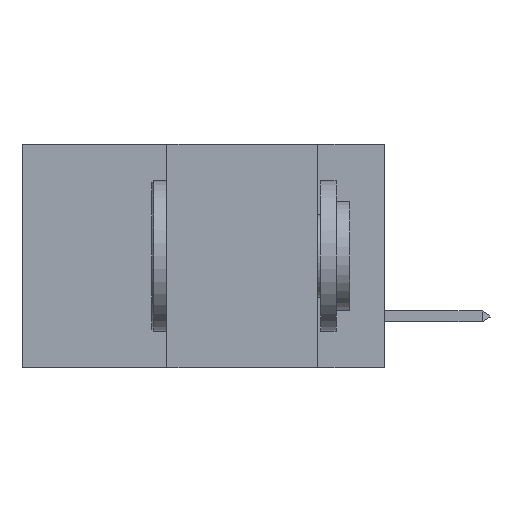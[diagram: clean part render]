
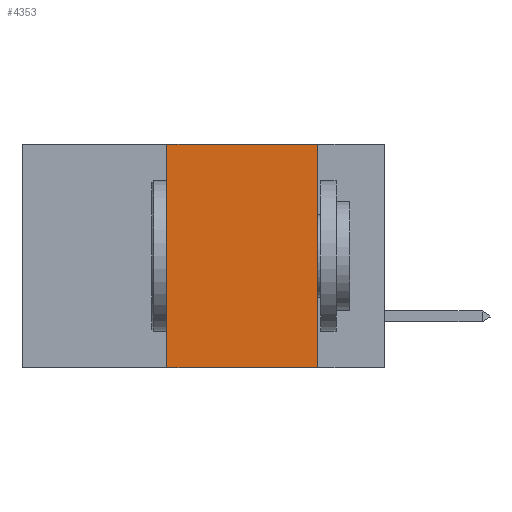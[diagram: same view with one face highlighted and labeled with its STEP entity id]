
A CAD part, left-side view. The second image highlights one B-rep face of the part: STEP entity #4353.
In plain terms, the highlighted planar face has unit normal (-1, 0, 0).
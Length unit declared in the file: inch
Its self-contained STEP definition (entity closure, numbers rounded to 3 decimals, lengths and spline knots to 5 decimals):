
#72 = CARTESIAN_POINT ( 'NONE',  ( 0., 0.11, -0.37 ) ) ;
#122 = CARTESIAN_POINT ( 'NONE',  ( 0., 0.36, -0.37 ) ) ;
#242 = CARTESIAN_POINT ( 'NONE',  ( 0., 0.36, 0. ) ) ;
#438 = CARTESIAN_POINT ( 'NONE',  ( 0., 0.11, 0. ) ) ;
#2073 = LINE ( 'NONE', #10217, #8807 ) ;
#2089 = ORIENTED_EDGE ( 'NONE', *, *, #7960, .F. ) ;
#2173 = PLANE ( 'NONE',  #8503 ) ;
#3237 = VECTOR ( 'NONE', #3608, 39.37008 ) ;
#3608 = DIRECTION ( 'NONE',  ( 0., -1., 0. ) ) ;
#3839 = LINE ( 'NONE', #12000, #12745 ) ;
#4127 = EDGE_CURVE ( 'NONE', #6710, #10587, #11072, .T. ) ;
#4353 = ADVANCED_FACE ( 'NONE', ( #7866 ), #2173, .F. ) ;
#4781 = VERTEX_POINT ( 'NONE', #72 ) ;
#5254 = VECTOR ( 'NONE', #5755, 39.37008 ) ;
#5564 = VERTEX_POINT ( 'NONE', #122 ) ;
#5755 = DIRECTION ( 'NONE',  ( 0., 0., -1. ) ) ;
#5961 = DIRECTION ( 'NONE',  ( 0., 0., -1. ) ) ;
#6324 = DIRECTION ( 'NONE',  ( 0., 0., 1. ) ) ;
#6710 = VERTEX_POINT ( 'NONE', #242 ) ;
#7640 = ORIENTED_EDGE ( 'NONE', *, *, #8305, .T. ) ;
#7866 = FACE_OUTER_BOUND ( 'NONE', #12494, .T. ) ;
#7960 = EDGE_CURVE ( 'NONE', #10587, #4781, #10149, .T. ) ;
#8305 = EDGE_CURVE ( 'NONE', #5564, #4781, #3839, .T. ) ;
#8353 = ORIENTED_EDGE ( 'NONE', *, *, #12231, .F. ) ;
#8503 = AXIS2_PLACEMENT_3D ( 'NONE', #10985, #11971, #5961 ) ;
#8807 = VECTOR ( 'NONE', #6324, 39.37008 ) ;
#9298 = DIRECTION ( 'NONE',  ( 0., -1., 0. ) ) ;
#9320 = CARTESIAN_POINT ( 'NONE',  ( 0., 0.11, 0. ) ) ;
#9481 = CARTESIAN_POINT ( 'NONE',  ( 0., 0.6, 0. ) ) ;
#9511 = ORIENTED_EDGE ( 'NONE', *, *, #4127, .F. ) ;
#10149 = LINE ( 'NONE', #438, #5254 ) ;
#10217 = CARTESIAN_POINT ( 'NONE',  ( 0., 0.36, 0. ) ) ;
#10587 = VERTEX_POINT ( 'NONE', #9320 ) ;
#10985 = CARTESIAN_POINT ( 'NONE',  ( 0., 0.6, 0. ) ) ;
#11072 = LINE ( 'NONE', #9481, #3237 ) ;
#11971 = DIRECTION ( 'NONE',  ( 1., 0., 0. ) ) ;
#12000 = CARTESIAN_POINT ( 'NONE',  ( 0., 0.6, -0.37 ) ) ;
#12231 = EDGE_CURVE ( 'NONE', #5564, #6710, #2073, .T. ) ;
#12494 = EDGE_LOOP ( 'NONE', ( #2089, #9511, #8353, #7640 ) ) ;
#12745 = VECTOR ( 'NONE', #9298, 39.37008 ) ;
